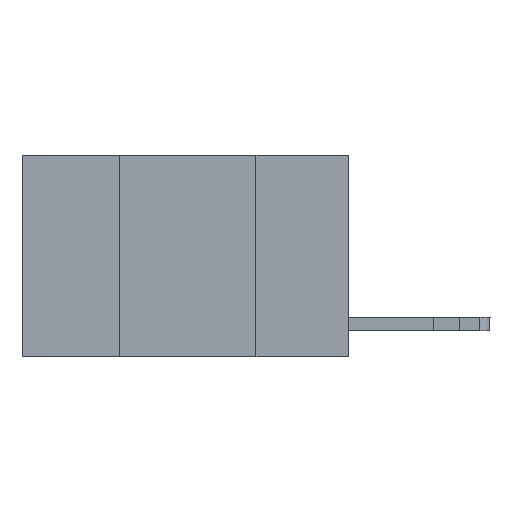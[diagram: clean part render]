
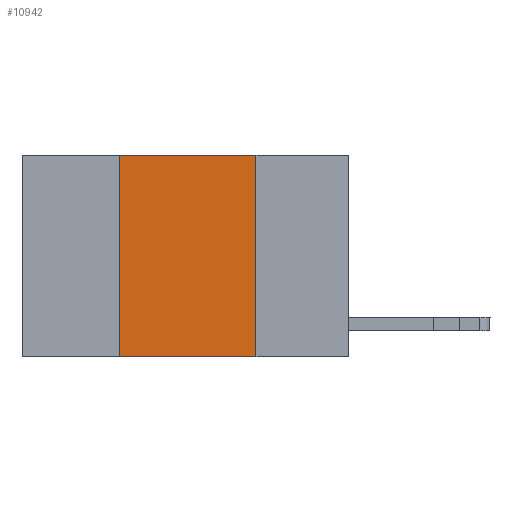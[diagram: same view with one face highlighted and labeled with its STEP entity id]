
A CAD part, left-side view. The second image highlights one B-rep face of the part: STEP entity #10942.
In plain terms, the highlighted planar face has unit normal (-1, 0, 0).
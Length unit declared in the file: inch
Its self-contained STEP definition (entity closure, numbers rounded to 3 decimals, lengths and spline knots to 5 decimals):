
#527 = EDGE_CURVE ( 'NONE', #16122, #16999, #16982, .T. ) ;
#1563 = ORIENTED_EDGE ( 'NONE', *, *, #527, .F. ) ;
#1636 = FACE_OUTER_BOUND ( 'NONE', #3336, .T. ) ;
#1979 = ORIENTED_EDGE ( 'NONE', *, *, #14310, .F. ) ;
#2441 = ORIENTED_EDGE ( 'NONE', *, *, #17278, .F. ) ;
#2532 = VERTEX_POINT ( 'NONE', #15129 ) ;
#2738 = CARTESIAN_POINT ( 'NONE',  ( 0., 0.6, 0. ) ) ;
#2793 = LINE ( 'NONE', #16358, #8814 ) ;
#2963 = CARTESIAN_POINT ( 'NONE',  ( 0., 0.6, 0. ) ) ;
#3131 = DIRECTION ( 'NONE',  ( 0., -1., 0. ) ) ;
#3297 = CARTESIAN_POINT ( 'NONE',  ( 0., 0.17, -0.37 ) ) ;
#3336 = EDGE_LOOP ( 'NONE', ( #1563, #1979, #2441, #16899 ) ) ;
#3365 = VECTOR ( 'NONE', #6614, 39.37008 ) ;
#4123 = DIRECTION ( 'NONE',  ( 0., 0., -1. ) ) ;
#4367 = DIRECTION ( 'NONE',  ( 0., -1., 0. ) ) ;
#6245 = LINE ( 'NONE', #14098, #13079 ) ;
#6614 = DIRECTION ( 'NONE',  ( 0., 0., -1. ) ) ;
#8184 = VECTOR ( 'NONE', #4367, 39.37008 ) ;
#8814 = VECTOR ( 'NONE', #13687, 39.37008 ) ;
#10942 = ADVANCED_FACE ( 'NONE', ( #1636 ), #10948, .F. ) ;
#10948 = PLANE ( 'NONE',  #14323 ) ;
#11506 = VERTEX_POINT ( 'NONE', #14771 ) ;
#12331 = DIRECTION ( 'NONE',  ( 1., 0., 0. ) ) ;
#13079 = VECTOR ( 'NONE', #3131, 39.37008 ) ;
#13488 = CARTESIAN_POINT ( 'NONE',  ( 0., 0.17, 0. ) ) ;
#13687 = DIRECTION ( 'NONE',  ( 0., 0., 1. ) ) ;
#14098 = CARTESIAN_POINT ( 'NONE',  ( 0., 0.6, -0.37 ) ) ;
#14310 = EDGE_CURVE ( 'NONE', #2532, #16122, #15846, .T. ) ;
#14323 = AXIS2_PLACEMENT_3D ( 'NONE', #2738, #12331, #4123 ) ;
#14771 = CARTESIAN_POINT ( 'NONE',  ( 0., 0.42, -0.37 ) ) ;
#14852 = CARTESIAN_POINT ( 'NONE',  ( 0., 0.17, 0. ) ) ;
#15129 = CARTESIAN_POINT ( 'NONE',  ( 0., 0.42, 0. ) ) ;
#15846 = LINE ( 'NONE', #2963, #8184 ) ;
#16122 = VERTEX_POINT ( 'NONE', #14852 ) ;
#16358 = CARTESIAN_POINT ( 'NONE',  ( 0., 0.42, 0. ) ) ;
#16392 = EDGE_CURVE ( 'NONE', #11506, #16999, #6245, .T. ) ;
#16899 = ORIENTED_EDGE ( 'NONE', *, *, #16392, .T. ) ;
#16982 = LINE ( 'NONE', #13488, #3365 ) ;
#16999 = VERTEX_POINT ( 'NONE', #3297 ) ;
#17278 = EDGE_CURVE ( 'NONE', #11506, #2532, #2793, .T. ) ;
